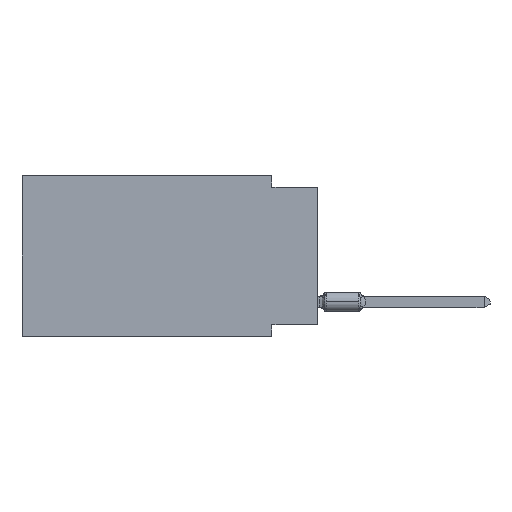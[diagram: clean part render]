
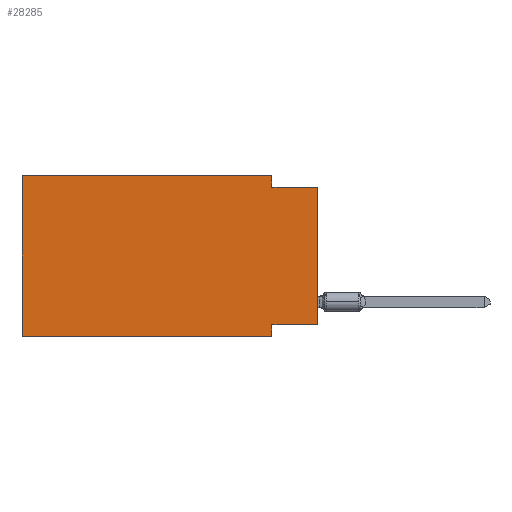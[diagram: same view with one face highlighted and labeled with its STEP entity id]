
A CAD part, left-side view. The second image highlights one B-rep face of the part: STEP entity #28285.
In plain terms, the highlighted planar face has unit normal (-1, 0, 0).
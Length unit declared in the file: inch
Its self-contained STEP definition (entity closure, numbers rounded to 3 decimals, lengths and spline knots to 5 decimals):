
#74 = CARTESIAN_POINT ( 'NONE',  ( 0., 0.645, -0.35 ) ) ;
#148 = DIRECTION ( 'NONE',  ( 1., 0., 0. ) ) ;
#1604 = ORIENTED_EDGE ( 'NONE', *, *, #1618, .F. ) ;
#1618 = EDGE_CURVE ( 'NONE', #15751, #24158, #14077, .T. ) ;
#2109 = VERTEX_POINT ( 'NONE', #29973 ) ;
#2320 = ORIENTED_EDGE ( 'NONE', *, *, #6255, .F. ) ;
#2366 = CARTESIAN_POINT ( 'NONE',  ( 0., 0.1, -0.325 ) ) ;
#2524 = EDGE_CURVE ( 'NONE', #19528, #2109, #14342, .T. ) ;
#3236 = FACE_OUTER_BOUND ( 'NONE', #15545, .T. ) ;
#4583 = DIRECTION ( 'NONE',  ( 0., -1., 0. ) ) ;
#5806 = EDGE_CURVE ( 'NONE', #2109, #19475, #21422, .T. ) ;
#6255 = EDGE_CURVE ( 'NONE', #24158, #21386, #36574, .T. ) ;
#7115 = VECTOR ( 'NONE', #33943, 39.37008 ) ;
#8150 = VECTOR ( 'NONE', #10188, 39.37008 ) ;
#8247 = ORIENTED_EDGE ( 'NONE', *, *, #31343, .F. ) ;
#8248 = DIRECTION ( 'NONE',  ( 0., 0., -1. ) ) ;
#8510 = CARTESIAN_POINT ( 'NONE',  ( 0., 0.645, 0. ) ) ;
#8701 = CARTESIAN_POINT ( 'NONE',  ( 0., 0.645, -0.35 ) ) ;
#10188 = DIRECTION ( 'NONE',  ( 0., 1., 0. ) ) ;
#14077 = LINE ( 'NONE', #38729, #8150 ) ;
#14323 = VECTOR ( 'NONE', #38971, 39.37008 ) ;
#14342 = LINE ( 'NONE', #26458, #14323 ) ;
#15545 = EDGE_LOOP ( 'NONE', ( #39985, #25390, #8247, #38420, #32286, #27045, #2320, #1604 ) ) ;
#15751 = VERTEX_POINT ( 'NONE', #39582 ) ;
#15758 = PLANE ( 'NONE',  #40222 ) ;
#16812 = CARTESIAN_POINT ( 'NONE',  ( 0., 0.1, 0. ) ) ;
#16898 = LINE ( 'NONE', #26724, #17949 ) ;
#17949 = VECTOR ( 'NONE', #4583, 39.37008 ) ;
#19096 = VECTOR ( 'NONE', #38446, 39.37008 ) ;
#19475 = VERTEX_POINT ( 'NONE', #20790 ) ;
#19528 = VERTEX_POINT ( 'NONE', #8701 ) ;
#20790 = CARTESIAN_POINT ( 'NONE',  ( 0., 0.1, 0. ) ) ;
#21386 = VERTEX_POINT ( 'NONE', #32442 ) ;
#21422 = LINE ( 'NONE', #8510, #7115 ) ;
#21544 = VECTOR ( 'NONE', #8248, 39.37008 ) ;
#23322 = DIRECTION ( 'NONE',  ( 0., 0., 1. ) ) ;
#24158 = VERTEX_POINT ( 'NONE', #2366 ) ;
#25116 = VECTOR ( 'NONE', #35683, 39.37008 ) ;
#25390 = ORIENTED_EDGE ( 'NONE', *, *, #35990, .F. ) ;
#25790 = EDGE_CURVE ( 'NONE', #19528, #21386, #38241, .T. ) ;
#26015 = LINE ( 'NONE', #29296, #32878 ) ;
#26458 = CARTESIAN_POINT ( 'NONE',  ( 0., 0.645, 0. ) ) ;
#26724 = CARTESIAN_POINT ( 'NONE',  ( 0., 0., -0.025 ) ) ;
#27045 = ORIENTED_EDGE ( 'NONE', *, *, #25790, .T. ) ;
#28275 = CARTESIAN_POINT ( 'NONE',  ( 0., 0.645, 0. ) ) ;
#28285 = ADVANCED_FACE ( 'NONE', ( #3236 ), #15758, .F. ) ;
#28920 = LINE ( 'NONE', #16812, #25116 ) ;
#29296 = CARTESIAN_POINT ( 'NONE',  ( 0., 0., 0. ) ) ;
#29371 = CARTESIAN_POINT ( 'NONE',  ( 0., 0., -0.025 ) ) ;
#29673 = EDGE_CURVE ( 'NONE', #15751, #30978, #26015, .T. ) ;
#29752 = CARTESIAN_POINT ( 'NONE',  ( 0., 0.1, -0.025 ) ) ;
#29973 = CARTESIAN_POINT ( 'NONE',  ( 0., 0.645, 0. ) ) ;
#30978 = VERTEX_POINT ( 'NONE', #29371 ) ;
#31343 = EDGE_CURVE ( 'NONE', #19475, #36481, #28920, .T. ) ;
#32286 = ORIENTED_EDGE ( 'NONE', *, *, #2524, .F. ) ;
#32442 = CARTESIAN_POINT ( 'NONE',  ( 0., 0.1, -0.35 ) ) ;
#32878 = VECTOR ( 'NONE', #23322, 39.37008 ) ;
#33943 = DIRECTION ( 'NONE',  ( 0., -1., 0. ) ) ;
#35683 = DIRECTION ( 'NONE',  ( 0., 0., -1. ) ) ;
#35990 = EDGE_CURVE ( 'NONE', #36481, #30978, #16898, .T. ) ;
#36362 = CARTESIAN_POINT ( 'NONE',  ( 0., 0.1, -0.35 ) ) ;
#36481 = VERTEX_POINT ( 'NONE', #29752 ) ;
#36574 = LINE ( 'NONE', #36362, #21544 ) ;
#37706 = DIRECTION ( 'NONE',  ( 0., 0., -1. ) ) ;
#38241 = LINE ( 'NONE', #74, #19096 ) ;
#38420 = ORIENTED_EDGE ( 'NONE', *, *, #5806, .F. ) ;
#38446 = DIRECTION ( 'NONE',  ( 0., -1., 0. ) ) ;
#38729 = CARTESIAN_POINT ( 'NONE',  ( 0., 0., -0.325 ) ) ;
#38971 = DIRECTION ( 'NONE',  ( 0., 0., 1. ) ) ;
#39582 = CARTESIAN_POINT ( 'NONE',  ( 0., 0., -0.325 ) ) ;
#39985 = ORIENTED_EDGE ( 'NONE', *, *, #29673, .T. ) ;
#40222 = AXIS2_PLACEMENT_3D ( 'NONE', #28275, #148, #37706 ) ;
